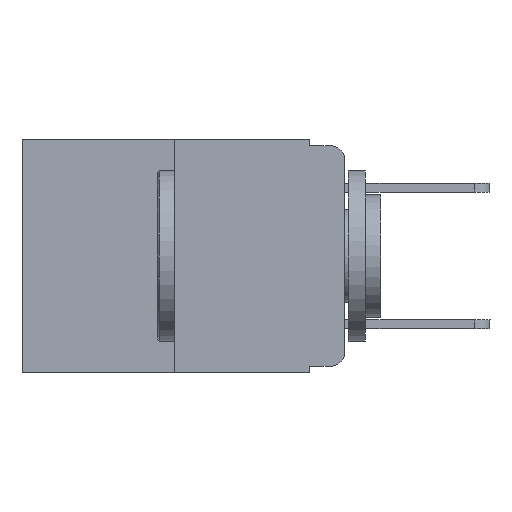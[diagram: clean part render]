
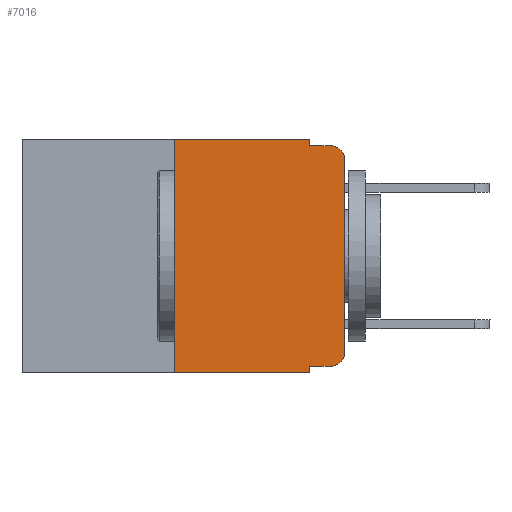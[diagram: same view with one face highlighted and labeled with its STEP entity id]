
A CAD part, left-side view. The second image highlights one B-rep face of the part: STEP entity #7016.
In plain terms, the highlighted planar face has unit normal (-1, 0, 0).
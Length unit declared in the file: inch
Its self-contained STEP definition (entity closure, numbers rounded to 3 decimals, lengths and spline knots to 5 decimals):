
#26 = ORIENTED_EDGE ( 'NONE', *, *, #13869, .T. ) ;
#82 = ORIENTED_EDGE ( 'NONE', *, *, #1084, .T. ) ;
#485 = EDGE_CURVE ( 'NONE', #20692, #15137, #4006, .T. ) ;
#572 = DIRECTION ( 'NONE',  ( -1., 0., 0. ) ) ;
#658 = CARTESIAN_POINT ( 'NONE',  ( 0., 0.473, 0. ) ) ;
#783 = CARTESIAN_POINT ( 'NONE',  ( 0., 0.02, -0.333 ) ) ;
#1034 = ORIENTED_EDGE ( 'NONE', *, *, #4719, .T. ) ;
#1084 = EDGE_CURVE ( 'NONE', #20871, #1894, #11204, .T. ) ;
#1114 = AXIS2_PLACEMENT_3D ( 'NONE', #658, #17855, #5421 ) ;
#1423 = CARTESIAN_POINT ( 'NONE',  ( 0., 0.051, -0.333 ) ) ;
#1697 = CARTESIAN_POINT ( 'NONE',  ( 0., 0.051, -0.01 ) ) ;
#1894 = VERTEX_POINT ( 'NONE', #6971 ) ;
#1909 = PLANE ( 'NONE',  #1114 ) ;
#2552 = VECTOR ( 'NONE', #15762, 39.37008 ) ;
#4006 = LINE ( 'NONE', #12502, #21939 ) ;
#4719 = EDGE_CURVE ( 'NONE', #6049, #19392, #13776, .T. ) ;
#4998 = ORIENTED_EDGE ( 'NONE', *, *, #485, .F. ) ;
#5374 = CARTESIAN_POINT ( 'NONE',  ( 0., 0.25, 0. ) ) ;
#5421 = DIRECTION ( 'NONE',  ( 0., 0., -1. ) ) ;
#5600 = ORIENTED_EDGE ( 'NONE', *, *, #8167, .F. ) ;
#5878 = VECTOR ( 'NONE', #12080, 39.37008 ) ;
#5945 = EDGE_CURVE ( 'NONE', #10455, #20871, #21882, .T. ) ;
#6049 = VERTEX_POINT ( 'NONE', #9834 ) ;
#6096 = LINE ( 'NONE', #7894, #7244 ) ;
#6213 = CARTESIAN_POINT ( 'NONE',  ( 0., 0.051, 0. ) ) ;
#6422 = VERTEX_POINT ( 'NONE', #20512 ) ;
#6809 = CARTESIAN_POINT ( 'NONE',  ( 0., 0., 0. ) ) ;
#6971 = CARTESIAN_POINT ( 'NONE',  ( 0., 0., -0.313 ) ) ;
#7016 = ADVANCED_FACE ( 'NONE', ( #12788 ), #1909, .F. ) ;
#7244 = VECTOR ( 'NONE', #13238, 39.37008 ) ;
#7474 = DIRECTION ( 'NONE',  ( 0., 0., -1. ) ) ;
#7894 = CARTESIAN_POINT ( 'NONE',  ( 0., 0.051, 0. ) ) ;
#8006 = ORIENTED_EDGE ( 'NONE', *, *, #10212, .F. ) ;
#8167 = EDGE_CURVE ( 'NONE', #8230, #20692, #6096, .T. ) ;
#8230 = VERTEX_POINT ( 'NONE', #6213 ) ;
#8893 = ORIENTED_EDGE ( 'NONE', *, *, #5945, .T. ) ;
#8984 = LINE ( 'NONE', #15857, #9323 ) ;
#9323 = VECTOR ( 'NONE', #14536, 39.37008 ) ;
#9834 = CARTESIAN_POINT ( 'NONE',  ( 0., 0.25, -0.343 ) ) ;
#10212 = EDGE_CURVE ( 'NONE', #6049, #21686, #19390, .T. ) ;
#10378 = EDGE_LOOP ( 'NONE', ( #26, #18015, #4998, #5600, #13002, #8006, #1034, #19240, #8893, #82 ) ) ;
#10394 = CARTESIAN_POINT ( 'NONE',  ( 0., 0.473, -0.343 ) ) ;
#10455 = VERTEX_POINT ( 'NONE', #22292 ) ;
#10821 = LINE ( 'NONE', #12186, #2552 ) ;
#11204 = CIRCLE ( 'NONE', #15515, 0.02 ) ;
#11497 = DIRECTION ( 'NONE',  ( 0., 0., -1. ) ) ;
#11694 = EDGE_CURVE ( 'NONE', #6422, #15137, #22184, .T. ) ;
#12080 = DIRECTION ( 'NONE',  ( 0., -1., 0. ) ) ;
#12186 = CARTESIAN_POINT ( 'NONE',  ( 0., 0.051, 0. ) ) ;
#12502 = CARTESIAN_POINT ( 'NONE',  ( 0., 0.051, -0.01 ) ) ;
#12788 = FACE_OUTER_BOUND ( 'NONE', #10378, .T. ) ;
#13002 = ORIENTED_EDGE ( 'NONE', *, *, #16522, .F. ) ;
#13238 = DIRECTION ( 'NONE',  ( 0., 0., -1. ) ) ;
#13280 = CARTESIAN_POINT ( 'NONE',  ( 0., 0.25, 0. ) ) ;
#13443 = DIRECTION ( 'NONE',  ( 0., -1., 0. ) ) ;
#13776 = LINE ( 'NONE', #10394, #5878 ) ;
#13869 = EDGE_CURVE ( 'NONE', #1894, #6422, #22285, .T. ) ;
#14536 = DIRECTION ( 'NONE',  ( 0., -1., 0. ) ) ;
#14651 = CARTESIAN_POINT ( 'NONE',  ( 0., 0.02, -0.03 ) ) ;
#15137 = VERTEX_POINT ( 'NONE', #22174 ) ;
#15515 = AXIS2_PLACEMENT_3D ( 'NONE', #17773, #572, #7474 ) ;
#15628 = DIRECTION ( 'NONE',  ( 0., 0., 1. ) ) ;
#15655 = CARTESIAN_POINT ( 'NONE',  ( 0., 0.051, -0.343 ) ) ;
#15762 = DIRECTION ( 'NONE',  ( 0., 0., -1. ) ) ;
#15857 = CARTESIAN_POINT ( 'NONE',  ( 0., 0.473, 0. ) ) ;
#16522 = EDGE_CURVE ( 'NONE', #21686, #8230, #8984, .T. ) ;
#17145 = AXIS2_PLACEMENT_3D ( 'NONE', #14651, #19961, #11497 ) ;
#17685 = DIRECTION ( 'NONE',  ( 0., 0., 1. ) ) ;
#17773 = CARTESIAN_POINT ( 'NONE',  ( 0., 0.02, -0.313 ) ) ;
#17855 = DIRECTION ( 'NONE',  ( 1., 0., 0. ) ) ;
#18015 = ORIENTED_EDGE ( 'NONE', *, *, #11694, .T. ) ;
#19240 = ORIENTED_EDGE ( 'NONE', *, *, #19458, .F. ) ;
#19382 = DIRECTION ( 'NONE',  ( 0., -1., 0. ) ) ;
#19390 = LINE ( 'NONE', #5374, #19813 ) ;
#19392 = VERTEX_POINT ( 'NONE', #15655 ) ;
#19458 = EDGE_CURVE ( 'NONE', #10455, #19392, #10821, .T. ) ;
#19813 = VECTOR ( 'NONE', #17685, 39.37008 ) ;
#19961 = DIRECTION ( 'NONE',  ( -1., 0., 0. ) ) ;
#20512 = CARTESIAN_POINT ( 'NONE',  ( 0., 0., -0.03 ) ) ;
#20692 = VERTEX_POINT ( 'NONE', #1697 ) ;
#20795 = VECTOR ( 'NONE', #13443, 39.37008 ) ;
#20871 = VERTEX_POINT ( 'NONE', #783 ) ;
#21686 = VERTEX_POINT ( 'NONE', #13280 ) ;
#21882 = LINE ( 'NONE', #1423, #20795 ) ;
#21883 = VECTOR ( 'NONE', #15628, 39.37008 ) ;
#21939 = VECTOR ( 'NONE', #19382, 39.37008 ) ;
#22174 = CARTESIAN_POINT ( 'NONE',  ( 0., 0.02, -0.01 ) ) ;
#22184 = CIRCLE ( 'NONE', #17145, 0.02 ) ;
#22285 = LINE ( 'NONE', #6809, #21883 ) ;
#22292 = CARTESIAN_POINT ( 'NONE',  ( 0., 0.051, -0.333 ) ) ;
